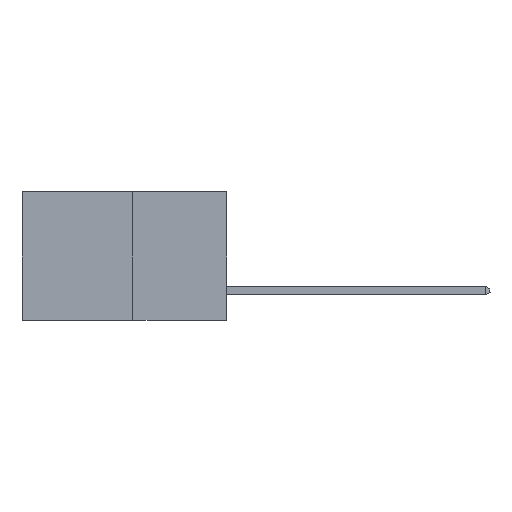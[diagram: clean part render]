
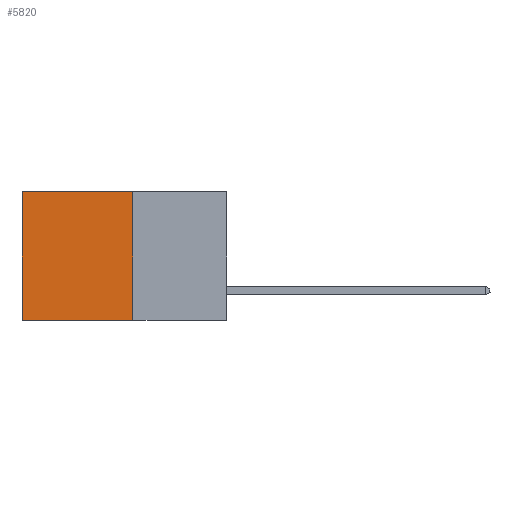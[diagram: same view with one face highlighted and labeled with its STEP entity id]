
A CAD part, left-side view. The second image highlights one B-rep face of the part: STEP entity #5820.
In plain terms, the highlighted planar face has unit normal (-1, 0, 0).
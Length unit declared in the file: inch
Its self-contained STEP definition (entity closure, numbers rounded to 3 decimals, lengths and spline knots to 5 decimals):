
#441 = DIRECTION ( 'NONE',  ( 0., 0., -1. ) ) ;
#478 = EDGE_CURVE ( 'NONE', #17224, #29170, #18074, .T. ) ;
#1238 = CARTESIAN_POINT ( 'NONE',  ( 0.277, 0.27, 0. ) ) ;
#2712 = CARTESIAN_POINT ( 'NONE',  ( 0.277, 0.59, -0.37 ) ) ;
#3732 = VECTOR ( 'NONE', #24804, 39.37008 ) ;
#5820 = ADVANCED_FACE ( 'NONE', ( #11289 ), #12021, .F. ) ;
#6060 = EDGE_LOOP ( 'NONE', ( #26308, #7588, #7217, #25143 ) ) ;
#7217 = ORIENTED_EDGE ( 'NONE', *, *, #21420, .F. ) ;
#7273 = CARTESIAN_POINT ( 'NONE',  ( 0.277, 0.27, -0.37 ) ) ;
#7588 = ORIENTED_EDGE ( 'NONE', *, *, #8011, .F. ) ;
#7808 = CARTESIAN_POINT ( 'NONE',  ( 0.277, 0.27, 0. ) ) ;
#7853 = DIRECTION ( 'NONE',  ( 0., 1., 0. ) ) ;
#8011 = EDGE_CURVE ( 'NONE', #22401, #12132, #10077, .T. ) ;
#10077 = LINE ( 'NONE', #7273, #3732 ) ;
#11289 = FACE_OUTER_BOUND ( 'NONE', #6060, .T. ) ;
#11946 = VECTOR ( 'NONE', #12137, 39.37008 ) ;
#12021 = PLANE ( 'NONE',  #18570 ) ;
#12132 = VERTEX_POINT ( 'NONE', #19288 ) ;
#12137 = DIRECTION ( 'NONE',  ( 0., 0., -1. ) ) ;
#13204 = VECTOR ( 'NONE', #441, 39.37008 ) ;
#15199 = CARTESIAN_POINT ( 'NONE',  ( 0.277, 0.59, 0. ) ) ;
#17224 = VERTEX_POINT ( 'NONE', #1238 ) ;
#18074 = LINE ( 'NONE', #7808, #24276 ) ;
#18570 = AXIS2_PLACEMENT_3D ( 'NONE', #29123, #29270, #29410 ) ;
#19165 = CARTESIAN_POINT ( 'NONE',  ( 0.277, 0.27, -0.37 ) ) ;
#19288 = CARTESIAN_POINT ( 'NONE',  ( 0.277, 0.59, -0.37 ) ) ;
#19376 = LINE ( 'NONE', #2712, #13204 ) ;
#21420 = EDGE_CURVE ( 'NONE', #17224, #22401, #29935, .T. ) ;
#22401 = VERTEX_POINT ( 'NONE', #24980 ) ;
#24276 = VECTOR ( 'NONE', #7853, 39.37008 ) ;
#24804 = DIRECTION ( 'NONE',  ( 0., 1., 0. ) ) ;
#24980 = CARTESIAN_POINT ( 'NONE',  ( 0.277, 0.27, -0.37 ) ) ;
#25143 = ORIENTED_EDGE ( 'NONE', *, *, #478, .T. ) ;
#25360 = EDGE_CURVE ( 'NONE', #29170, #12132, #19376, .T. ) ;
#26308 = ORIENTED_EDGE ( 'NONE', *, *, #25360, .T. ) ;
#29123 = CARTESIAN_POINT ( 'NONE',  ( 0.277, 0.27, -0.37 ) ) ;
#29170 = VERTEX_POINT ( 'NONE', #15199 ) ;
#29270 = DIRECTION ( 'NONE',  ( 1., 0., 0. ) ) ;
#29410 = DIRECTION ( 'NONE',  ( 0., 0., -1. ) ) ;
#29935 = LINE ( 'NONE', #19165, #11946 ) ;
